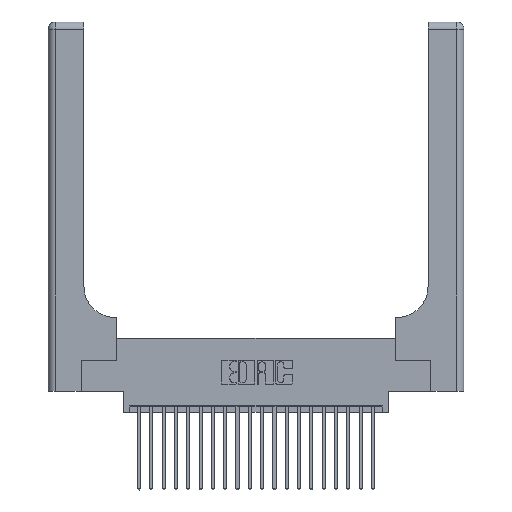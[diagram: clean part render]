
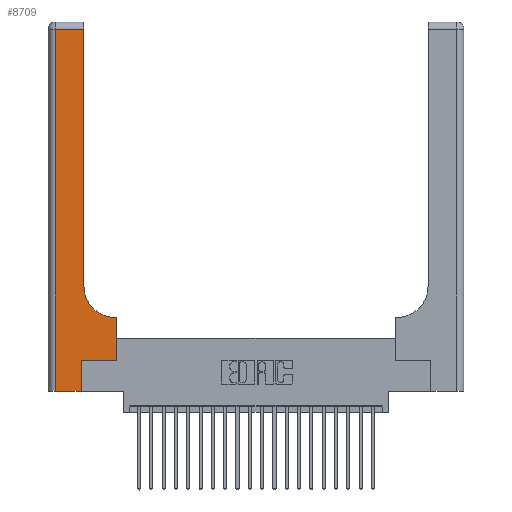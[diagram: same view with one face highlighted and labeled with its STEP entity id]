
A CAD part, top view. The second image highlights one B-rep face of the part: STEP entity #8709.
In plain terms, the highlighted planar face has unit normal (0, 0, 1).
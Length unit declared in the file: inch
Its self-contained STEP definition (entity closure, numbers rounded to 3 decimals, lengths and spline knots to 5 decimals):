
#18 = ORIENTED_EDGE ( 'NONE', *, *, #15405, .T. ) ;
#34 = CARTESIAN_POINT ( 'NONE',  ( 0.5585, 0.6, 0.37 ) ) ;
#136 = EDGE_CURVE ( 'NONE', #17283, #22425, #8824, .T. ) ;
#447 = CARTESIAN_POINT ( 'NONE',  ( 0.269, 0.25, 0.37 ) ) ;
#1055 = CARTESIAN_POINT ( 'NONE',  ( 0.269, 0., 0.37 ) ) ;
#1284 = VERTEX_POINT ( 'NONE', #5325 ) ;
#1294 = VECTOR ( 'NONE', #8607, 39.37008 ) ;
#1308 = CARTESIAN_POINT ( 'NONE',  ( 0.06, 0., 0.37 ) ) ;
#2297 = CIRCLE ( 'NONE', #19460, 0.25 ) ;
#2412 = CARTESIAN_POINT ( 'NONE',  ( 0.2915, 0.6, 0.37 ) ) ;
#2604 = VECTOR ( 'NONE', #15532, 39.37008 ) ;
#2762 = ORIENTED_EDGE ( 'NONE', *, *, #12763, .T. ) ;
#2838 = ORIENTED_EDGE ( 'NONE', *, *, #5625, .T. ) ;
#2871 = CARTESIAN_POINT ( 'NONE',  ( 0.2915, 2.94, 0.37 ) ) ;
#3272 = VERTEX_POINT ( 'NONE', #10707 ) ;
#3303 = EDGE_LOOP ( 'NONE', ( #3907, #2762, #18, #11679, #2838, #21827, #20658, #17383, #18086 ) ) ;
#3907 = ORIENTED_EDGE ( 'NONE', *, *, #136, .T. ) ;
#4051 = LINE ( 'NONE', #19364, #22554 ) ;
#4889 = LINE ( 'NONE', #20917, #9243 ) ;
#5253 = EDGE_CURVE ( 'NONE', #12624, #17283, #2297, .T. ) ;
#5325 = CARTESIAN_POINT ( 'NONE',  ( 0.06, 2.94, 0.37 ) ) ;
#5567 = EDGE_CURVE ( 'NONE', #8676, #5721, #10738, .T. ) ;
#5625 = EDGE_CURVE ( 'NONE', #5721, #3272, #19960, .T. ) ;
#5677 = EDGE_CURVE ( 'NONE', #3272, #10621, #11882, .T. ) ;
#5721 = VERTEX_POINT ( 'NONE', #19077 ) ;
#6082 = DIRECTION ( 'NONE',  ( 0., 1., 0. ) ) ;
#7268 = VECTOR ( 'NONE', #17143, 39.37008 ) ;
#8283 = CARTESIAN_POINT ( 'NONE',  ( 0.2915, 3., 0.37 ) ) ;
#8607 = DIRECTION ( 'NONE',  ( 0., -1., 0. ) ) ;
#8676 = VERTEX_POINT ( 'NONE', #1308 ) ;
#8709 = ADVANCED_FACE ( 'NONE', ( #20990 ), #22161, .F. ) ;
#8725 = DIRECTION ( 'NONE',  ( 1., 0., 0. ) ) ;
#8824 = LINE ( 'NONE', #8283, #22976 ) ;
#9243 = VECTOR ( 'NONE', #15281, 39.37008 ) ;
#9561 = VECTOR ( 'NONE', #22109, 39.37008 ) ;
#10621 = VERTEX_POINT ( 'NONE', #11345 ) ;
#10639 = CARTESIAN_POINT ( 'NONE',  ( 0.5415, 0.6, 0.37 ) ) ;
#10707 = CARTESIAN_POINT ( 'NONE',  ( 0.269, 0.25, 0.37 ) ) ;
#10738 = LINE ( 'NONE', #23662, #9561 ) ;
#11013 = DIRECTION ( 'NONE',  ( -1., 0., 0. ) ) ;
#11043 = LINE ( 'NONE', #2412, #7268 ) ;
#11345 = CARTESIAN_POINT ( 'NONE',  ( 0.5585, 0.25, 0.37 ) ) ;
#11679 = ORIENTED_EDGE ( 'NONE', *, *, #5567, .T. ) ;
#11810 = EDGE_CURVE ( 'NONE', #10621, #19652, #4051, .T. ) ;
#11882 = LINE ( 'NONE', #447, #2604 ) ;
#12599 = LINE ( 'NONE', #19570, #1294 ) ;
#12624 = VERTEX_POINT ( 'NONE', #10639 ) ;
#12763 = EDGE_CURVE ( 'NONE', #22425, #1284, #4889, .T. ) ;
#14646 = AXIS2_PLACEMENT_3D ( 'NONE', #16528, #22086, #11013 ) ;
#15281 = DIRECTION ( 'NONE',  ( -1., 0., 0. ) ) ;
#15405 = EDGE_CURVE ( 'NONE', #1284, #8676, #12599, .T. ) ;
#15532 = DIRECTION ( 'NONE',  ( 1., 0., 0. ) ) ;
#16528 = CARTESIAN_POINT ( 'NONE',  ( 0., 3., 0.37 ) ) ;
#17143 = DIRECTION ( 'NONE',  ( -1., 0., 0. ) ) ;
#17283 = VERTEX_POINT ( 'NONE', #18163 ) ;
#17383 = ORIENTED_EDGE ( 'NONE', *, *, #18239, .T. ) ;
#17652 = VECTOR ( 'NONE', #23325, 39.37008 ) ;
#18062 = CARTESIAN_POINT ( 'NONE',  ( 0.5415, 0.85, 0.37 ) ) ;
#18086 = ORIENTED_EDGE ( 'NONE', *, *, #5253, .T. ) ;
#18163 = CARTESIAN_POINT ( 'NONE',  ( 0.2915, 0.85, 0.37 ) ) ;
#18239 = EDGE_CURVE ( 'NONE', #19652, #12624, #11043, .T. ) ;
#19077 = CARTESIAN_POINT ( 'NONE',  ( 0.269, 0., 0.37 ) ) ;
#19364 = CARTESIAN_POINT ( 'NONE',  ( 0.5585, 0.25, 0.37 ) ) ;
#19460 = AXIS2_PLACEMENT_3D ( 'NONE', #18062, #19759, #8725 ) ;
#19570 = CARTESIAN_POINT ( 'NONE',  ( 0.06, 3., 0.37 ) ) ;
#19652 = VERTEX_POINT ( 'NONE', #34 ) ;
#19759 = DIRECTION ( 'NONE',  ( 0., 0., -1. ) ) ;
#19960 = LINE ( 'NONE', #1055, #17652 ) ;
#20658 = ORIENTED_EDGE ( 'NONE', *, *, #11810, .T. ) ;
#20917 = CARTESIAN_POINT ( 'NONE',  ( 0., 2.94, 0.37 ) ) ;
#20990 = FACE_OUTER_BOUND ( 'NONE', #3303, .T. ) ;
#21137 = DIRECTION ( 'NONE',  ( 0., 1., 0. ) ) ;
#21827 = ORIENTED_EDGE ( 'NONE', *, *, #5677, .T. ) ;
#22086 = DIRECTION ( 'NONE',  ( 0., 0., -1. ) ) ;
#22109 = DIRECTION ( 'NONE',  ( 1., 0., 0. ) ) ;
#22161 = PLANE ( 'NONE',  #14646 ) ;
#22425 = VERTEX_POINT ( 'NONE', #2871 ) ;
#22554 = VECTOR ( 'NONE', #21137, 39.37008 ) ;
#22976 = VECTOR ( 'NONE', #6082, 39.37008 ) ;
#23325 = DIRECTION ( 'NONE',  ( 0., 1., 0. ) ) ;
#23662 = CARTESIAN_POINT ( 'NONE',  ( 0., 0., 0.37 ) ) ;
